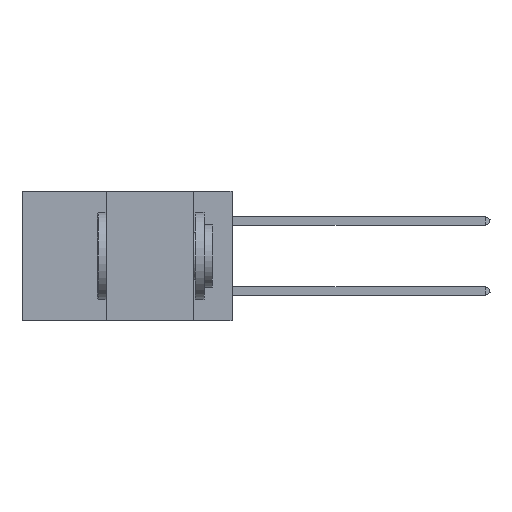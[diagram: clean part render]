
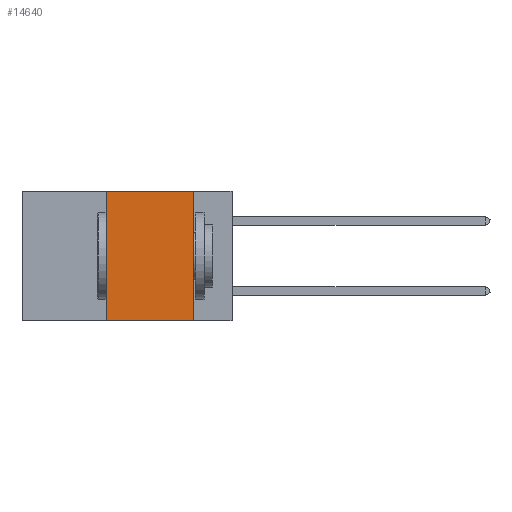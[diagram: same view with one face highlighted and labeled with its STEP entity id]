
A CAD part, left-side view. The second image highlights one B-rep face of the part: STEP entity #14640.
In plain terms, the highlighted planar face has unit normal (-1, 0, 0).
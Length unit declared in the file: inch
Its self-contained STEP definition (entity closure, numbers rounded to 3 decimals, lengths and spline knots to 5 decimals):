
#2081 = CARTESIAN_POINT ( 'NONE',  ( 0., 0.6, 0. ) ) ;
#2543 = CARTESIAN_POINT ( 'NONE',  ( 0., 0.36, 0. ) ) ;
#2710 = DIRECTION ( 'NONE',  ( 0., 0., 1. ) ) ;
#3728 = VERTEX_POINT ( 'NONE', #22177 ) ;
#4127 = EDGE_CURVE ( 'NONE', #42731, #10669, #46476, .T. ) ;
#6208 = LINE ( 'NONE', #2081, #44908 ) ;
#6672 = DIRECTION ( 'NONE',  ( 1., 0., 0. ) ) ;
#9511 = LINE ( 'NONE', #2543, #37651 ) ;
#10322 = CARTESIAN_POINT ( 'NONE',  ( 0., 0.11, -0.37 ) ) ;
#10669 = VERTEX_POINT ( 'NONE', #10322 ) ;
#10772 = DIRECTION ( 'NONE',  ( 0., 0., -1. ) ) ;
#12487 = EDGE_CURVE ( 'NONE', #3728, #42731, #6208, .T. ) ;
#12644 = CARTESIAN_POINT ( 'NONE',  ( 0., 0.6, -0.37 ) ) ;
#12649 = DIRECTION ( 'NONE',  ( 0., 0., -1. ) ) ;
#14417 = ORIENTED_EDGE ( 'NONE', *, *, #4127, .F. ) ;
#14640 = ADVANCED_FACE ( 'NONE', ( #25372 ), #44359, .F. ) ;
#15634 = CARTESIAN_POINT ( 'NONE',  ( 0., 0.11, 0. ) ) ;
#16128 = ORIENTED_EDGE ( 'NONE', *, *, #20896, .F. ) ;
#18232 = VERTEX_POINT ( 'NONE', #41932 ) ;
#19792 = CARTESIAN_POINT ( 'NONE',  ( 0., 0.11, 0. ) ) ;
#20896 = EDGE_CURVE ( 'NONE', #18232, #3728, #9511, .T. ) ;
#22177 = CARTESIAN_POINT ( 'NONE',  ( 0., 0.36, 0. ) ) ;
#25372 = FACE_OUTER_BOUND ( 'NONE', #48229, .T. ) ;
#30678 = VECTOR ( 'NONE', #12649, 39.37008 ) ;
#33988 = ORIENTED_EDGE ( 'NONE', *, *, #12487, .F. ) ;
#34958 = DIRECTION ( 'NONE',  ( 0., -1., 0. ) ) ;
#35690 = DIRECTION ( 'NONE',  ( 0., -1., 0. ) ) ;
#36723 = VECTOR ( 'NONE', #34958, 39.37008 ) ;
#37651 = VECTOR ( 'NONE', #2710, 39.37008 ) ;
#41932 = CARTESIAN_POINT ( 'NONE',  ( 0., 0.36, -0.37 ) ) ;
#42731 = VERTEX_POINT ( 'NONE', #19792 ) ;
#43876 = ORIENTED_EDGE ( 'NONE', *, *, #46852, .T. ) ;
#44263 = AXIS2_PLACEMENT_3D ( 'NONE', #48140, #6672, #10772 ) ;
#44359 = PLANE ( 'NONE',  #44263 ) ;
#44908 = VECTOR ( 'NONE', #35690, 39.37008 ) ;
#46476 = LINE ( 'NONE', #15634, #30678 ) ;
#46651 = LINE ( 'NONE', #12644, #36723 ) ;
#46852 = EDGE_CURVE ( 'NONE', #18232, #10669, #46651, .T. ) ;
#48140 = CARTESIAN_POINT ( 'NONE',  ( 0., 0.6, 0. ) ) ;
#48229 = EDGE_LOOP ( 'NONE', ( #14417, #33988, #16128, #43876 ) ) ;
